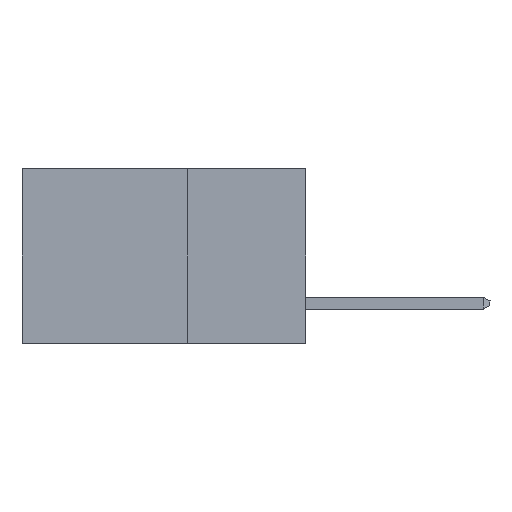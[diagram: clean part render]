
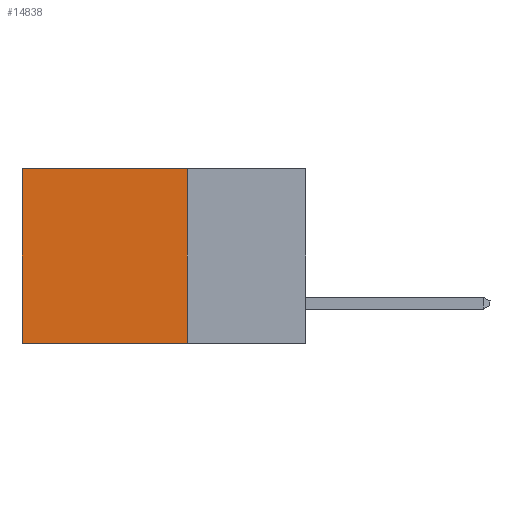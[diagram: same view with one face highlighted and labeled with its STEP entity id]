
A CAD part, left-side view. The second image highlights one B-rep face of the part: STEP entity #14838.
In plain terms, the highlighted planar face has unit normal (-1, 0, 0).
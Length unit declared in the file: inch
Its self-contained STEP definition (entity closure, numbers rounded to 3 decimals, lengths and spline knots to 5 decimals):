
#346 = LINE ( 'NONE', #3230, #3324 ) ;
#738 = VECTOR ( 'NONE', #25682, 39.37008 ) ;
#1947 = ORIENTED_EDGE ( 'NONE', *, *, #12753, .F. ) ;
#2602 = VECTOR ( 'NONE', #26741, 39.37008 ) ;
#3230 = CARTESIAN_POINT ( 'NONE',  ( 0.298, 0.25, 0. ) ) ;
#3324 = VECTOR ( 'NONE', #13845, 39.37008 ) ;
#3402 = VECTOR ( 'NONE', #18290, 39.37008 ) ;
#4096 = DIRECTION ( 'NONE',  ( 0., 0., -1. ) ) ;
#6383 = LINE ( 'NONE', #12980, #738 ) ;
#8390 = AXIS2_PLACEMENT_3D ( 'NONE', #16922, #23139, #4096 ) ;
#9190 = CARTESIAN_POINT ( 'NONE',  ( 0.298, 0.6, 0. ) ) ;
#12638 = PLANE ( 'NONE',  #8390 ) ;
#12753 = EDGE_CURVE ( 'NONE', #16436, #24589, #14619, .T. ) ;
#12980 = CARTESIAN_POINT ( 'NONE',  ( 0.298, 0.6, 0. ) ) ;
#13297 = FACE_OUTER_BOUND ( 'NONE', #21268, .T. ) ;
#13845 = DIRECTION ( 'NONE',  ( 0., 0., -1. ) ) ;
#14446 = EDGE_CURVE ( 'NONE', #24373, #14550, #17428, .T. ) ;
#14550 = VERTEX_POINT ( 'NONE', #9190 ) ;
#14619 = LINE ( 'NONE', #26927, #2602 ) ;
#14838 = ADVANCED_FACE ( 'NONE', ( #13297 ), #12638, .F. ) ;
#15343 = CARTESIAN_POINT ( 'NONE',  ( 0.298, 0.25, -0.37 ) ) ;
#16211 = ORIENTED_EDGE ( 'NONE', *, *, #14446, .T. ) ;
#16436 = VERTEX_POINT ( 'NONE', #15343 ) ;
#16922 = CARTESIAN_POINT ( 'NONE',  ( 0.298, 0.25, 0. ) ) ;
#17428 = LINE ( 'NONE', #22818, #3402 ) ;
#18290 = DIRECTION ( 'NONE',  ( 0., 1., 0. ) ) ;
#18860 = EDGE_CURVE ( 'NONE', #14550, #24589, #6383, .T. ) ;
#21165 = CARTESIAN_POINT ( 'NONE',  ( 0.298, 0.6, -0.37 ) ) ;
#21268 = EDGE_LOOP ( 'NONE', ( #22570, #1947, #26567, #16211 ) ) ;
#22570 = ORIENTED_EDGE ( 'NONE', *, *, #18860, .T. ) ;
#22818 = CARTESIAN_POINT ( 'NONE',  ( 0.298, 0.25, 0. ) ) ;
#23139 = DIRECTION ( 'NONE',  ( 1., 0., 0. ) ) ;
#24343 = CARTESIAN_POINT ( 'NONE',  ( 0.298, 0.25, 0. ) ) ;
#24373 = VERTEX_POINT ( 'NONE', #24343 ) ;
#24589 = VERTEX_POINT ( 'NONE', #21165 ) ;
#25682 = DIRECTION ( 'NONE',  ( 0., 0., -1. ) ) ;
#26567 = ORIENTED_EDGE ( 'NONE', *, *, #27142, .F. ) ;
#26741 = DIRECTION ( 'NONE',  ( 0., 1., 0. ) ) ;
#26927 = CARTESIAN_POINT ( 'NONE',  ( 0.298, 0.25, -0.37 ) ) ;
#27142 = EDGE_CURVE ( 'NONE', #24373, #16436, #346, .T. ) ;
